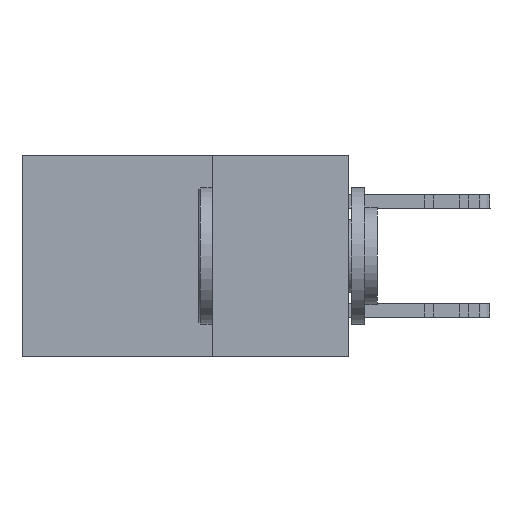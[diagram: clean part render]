
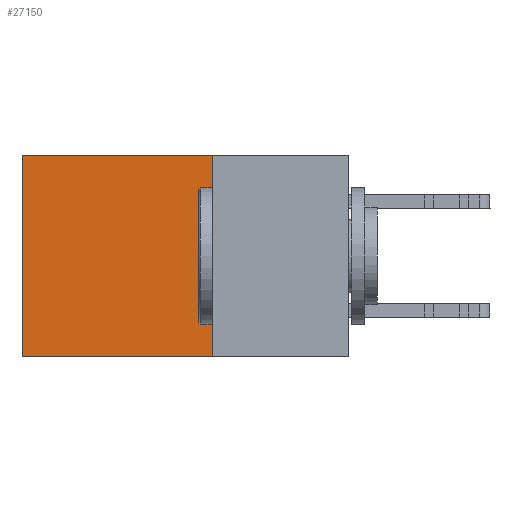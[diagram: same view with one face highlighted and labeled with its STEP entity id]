
A CAD part, left-side view. The second image highlights one B-rep face of the part: STEP entity #27150.
In plain terms, the highlighted planar face has unit normal (-1, 0, 0).
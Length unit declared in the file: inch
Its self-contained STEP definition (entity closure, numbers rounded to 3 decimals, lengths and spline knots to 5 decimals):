
#82 = CARTESIAN_POINT ( 'NONE',  ( 0.298, 0.25, 0. ) ) ;
#2184 = DIRECTION ( 'NONE',  ( 0., 0., -1. ) ) ;
#2416 = DIRECTION ( 'NONE',  ( 0., 0., -1. ) ) ;
#3286 = EDGE_LOOP ( 'NONE', ( #29247, #23745, #6770, #3544 ) ) ;
#3544 = ORIENTED_EDGE ( 'NONE', *, *, #23173, .T. ) ;
#5069 = VERTEX_POINT ( 'NONE', #9220 ) ;
#5221 = DIRECTION ( 'NONE',  ( 0., 0., -1. ) ) ;
#5243 = EDGE_CURVE ( 'NONE', #5069, #10803, #21271, .T. ) ;
#5875 = CARTESIAN_POINT ( 'NONE',  ( 0.298, 0.25, -0.37 ) ) ;
#6538 = CARTESIAN_POINT ( 'NONE',  ( 0.298, 0.6, 0. ) ) ;
#6770 = ORIENTED_EDGE ( 'NONE', *, *, #5243, .F. ) ;
#7241 = AXIS2_PLACEMENT_3D ( 'NONE', #82, #15979, #2416 ) ;
#7415 = CARTESIAN_POINT ( 'NONE',  ( 0.298, 0.25, 0. ) ) ;
#8435 = VERTEX_POINT ( 'NONE', #22611 ) ;
#9220 = CARTESIAN_POINT ( 'NONE',  ( 0.298, 0.25, 0. ) ) ;
#10243 = VERTEX_POINT ( 'NONE', #6538 ) ;
#10803 = VERTEX_POINT ( 'NONE', #16064 ) ;
#11826 = EDGE_CURVE ( 'NONE', #10803, #8435, #16799, .T. ) ;
#13534 = CARTESIAN_POINT ( 'NONE',  ( 0.298, 0.6, 0. ) ) ;
#13560 = VECTOR ( 'NONE', #25746, 39.37008 ) ;
#15367 = VECTOR ( 'NONE', #5221, 39.37008 ) ;
#15979 = DIRECTION ( 'NONE',  ( 1., 0., 0. ) ) ;
#16064 = CARTESIAN_POINT ( 'NONE',  ( 0.298, 0.25, -0.37 ) ) ;
#16799 = LINE ( 'NONE', #5875, #17477 ) ;
#17477 = VECTOR ( 'NONE', #21578, 39.37008 ) ;
#19186 = LINE ( 'NONE', #13534, #23815 ) ;
#19431 = LINE ( 'NONE', #23500, #13560 ) ;
#19919 = EDGE_CURVE ( 'NONE', #10243, #8435, #19186, .T. ) ;
#20217 = FACE_OUTER_BOUND ( 'NONE', #3286, .T. ) ;
#21271 = LINE ( 'NONE', #7415, #15367 ) ;
#21578 = DIRECTION ( 'NONE',  ( 0., 1., 0. ) ) ;
#22611 = CARTESIAN_POINT ( 'NONE',  ( 0.298, 0.6, -0.37 ) ) ;
#22625 = PLANE ( 'NONE',  #7241 ) ;
#23173 = EDGE_CURVE ( 'NONE', #5069, #10243, #19431, .T. ) ;
#23500 = CARTESIAN_POINT ( 'NONE',  ( 0.298, 0.25, 0. ) ) ;
#23745 = ORIENTED_EDGE ( 'NONE', *, *, #11826, .F. ) ;
#23815 = VECTOR ( 'NONE', #2184, 39.37008 ) ;
#25746 = DIRECTION ( 'NONE',  ( 0., 1., 0. ) ) ;
#27150 = ADVANCED_FACE ( 'NONE', ( #20217 ), #22625, .F. ) ;
#29247 = ORIENTED_EDGE ( 'NONE', *, *, #19919, .T. ) ;
